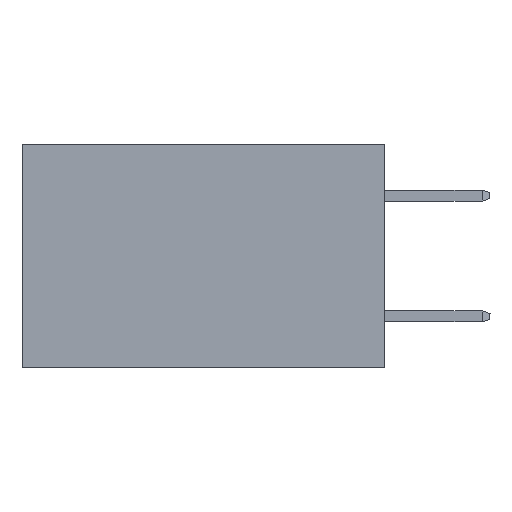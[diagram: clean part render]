
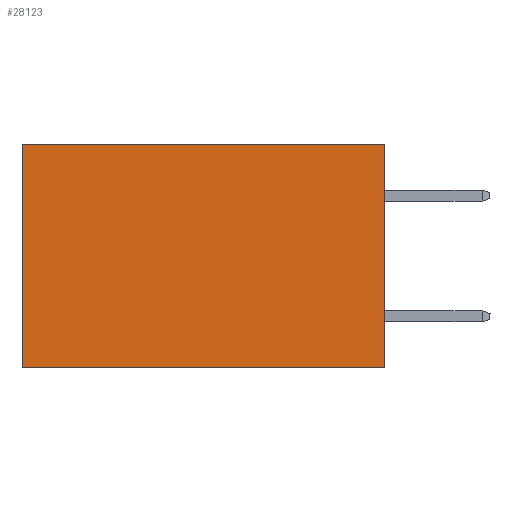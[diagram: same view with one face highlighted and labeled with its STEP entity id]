
A CAD part, left-side view. The second image highlights one B-rep face of the part: STEP entity #28123.
In plain terms, the highlighted planar face has unit normal (-1, 0, 0).
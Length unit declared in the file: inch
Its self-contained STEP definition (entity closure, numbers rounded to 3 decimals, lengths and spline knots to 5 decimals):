
#518 = ORIENTED_EDGE ( 'NONE', *, *, #26134, .T. ) ;
#1232 = DIRECTION ( 'NONE',  ( 0., 0., -1. ) ) ;
#2108 = CARTESIAN_POINT ( 'NONE',  ( 0.298, 0., -0.37 ) ) ;
#2343 = DIRECTION ( 'NONE',  ( 0., 1., 0. ) ) ;
#5377 = CARTESIAN_POINT ( 'NONE',  ( 0.298, 0.6, 0. ) ) ;
#7242 = CARTESIAN_POINT ( 'NONE',  ( 0.298, 0.6, -0.37 ) ) ;
#7740 = VECTOR ( 'NONE', #21723, 39.37008 ) ;
#9192 = LINE ( 'NONE', #14771, #7740 ) ;
#9493 = ORIENTED_EDGE ( 'NONE', *, *, #14561, .T. ) ;
#10596 = VECTOR ( 'NONE', #17314, 39.37008 ) ;
#11044 = DIRECTION ( 'NONE',  ( 0., 0., -1. ) ) ;
#12782 = CARTESIAN_POINT ( 'NONE',  ( 0.298, 0., 0. ) ) ;
#14404 = ORIENTED_EDGE ( 'NONE', *, *, #26379, .F. ) ;
#14561 = EDGE_CURVE ( 'NONE', #22188, #18274, #28854, .T. ) ;
#14771 = CARTESIAN_POINT ( 'NONE',  ( 0.298, 0.6, 0. ) ) ;
#15084 = DIRECTION ( 'NONE',  ( 1., 0., 0. ) ) ;
#17314 = DIRECTION ( 'NONE',  ( 0., 1., 0. ) ) ;
#17629 = EDGE_LOOP ( 'NONE', ( #518, #23507, #14404, #9493 ) ) ;
#18274 = VERTEX_POINT ( 'NONE', #5377 ) ;
#18417 = CARTESIAN_POINT ( 'NONE',  ( 0.298, 0., -0.37 ) ) ;
#18911 = VECTOR ( 'NONE', #11044, 39.37008 ) ;
#20107 = AXIS2_PLACEMENT_3D ( 'NONE', #12782, #15084, #1232 ) ;
#20173 = CARTESIAN_POINT ( 'NONE',  ( 0.298, 0., 0. ) ) ;
#21302 = VECTOR ( 'NONE', #2343, 39.37008 ) ;
#21723 = DIRECTION ( 'NONE',  ( 0., 0., -1. ) ) ;
#22188 = VERTEX_POINT ( 'NONE', #27368 ) ;
#22365 = VERTEX_POINT ( 'NONE', #7242 ) ;
#22983 = EDGE_CURVE ( 'NONE', #23616, #22365, #27389, .T. ) ;
#23507 = ORIENTED_EDGE ( 'NONE', *, *, #22983, .F. ) ;
#23616 = VERTEX_POINT ( 'NONE', #2108 ) ;
#25031 = LINE ( 'NONE', #20173, #18911 ) ;
#26134 = EDGE_CURVE ( 'NONE', #18274, #22365, #9192, .T. ) ;
#26379 = EDGE_CURVE ( 'NONE', #22188, #23616, #25031, .T. ) ;
#26796 = FACE_OUTER_BOUND ( 'NONE', #17629, .T. ) ;
#27368 = CARTESIAN_POINT ( 'NONE',  ( 0.298, 0., 0. ) ) ;
#27389 = LINE ( 'NONE', #18417, #21302 ) ;
#28123 = ADVANCED_FACE ( 'NONE', ( #26796 ), #28773, .F. ) ;
#28696 = CARTESIAN_POINT ( 'NONE',  ( 0.298, 0., 0. ) ) ;
#28773 = PLANE ( 'NONE',  #20107 ) ;
#28854 = LINE ( 'NONE', #28696, #10596 ) ;
